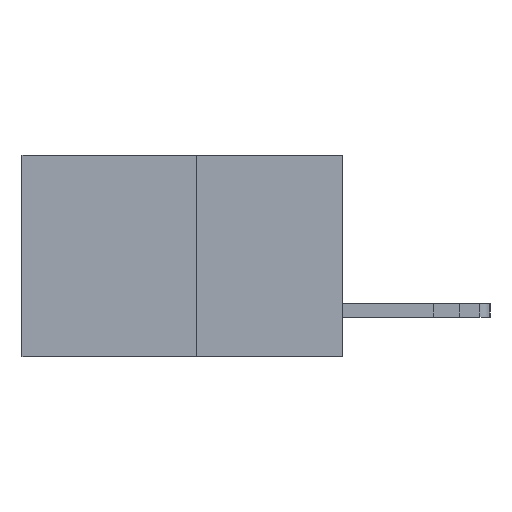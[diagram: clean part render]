
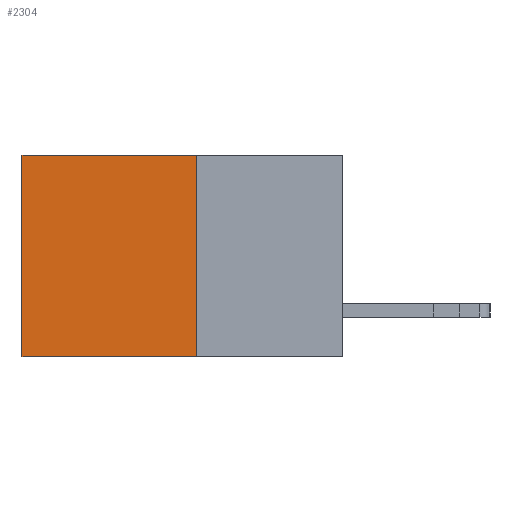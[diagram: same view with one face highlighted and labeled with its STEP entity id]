
A CAD part, left-side view. The second image highlights one B-rep face of the part: STEP entity #2304.
In plain terms, the highlighted planar face has unit normal (-1, 0, 0).
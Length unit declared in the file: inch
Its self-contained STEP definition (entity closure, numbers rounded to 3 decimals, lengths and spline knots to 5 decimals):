
#92 = EDGE_CURVE ( 'NONE', #1988, #14659, #19713, .T. ) ;
#217 = AXIS2_PLACEMENT_3D ( 'NONE', #9727, #699, #9771 ) ;
#699 = DIRECTION ( 'NONE',  ( 1., 0., 0. ) ) ;
#1071 = CARTESIAN_POINT ( 'NONE',  ( 0.277, 0.59, -0.37 ) ) ;
#1251 = EDGE_CURVE ( 'NONE', #15106, #1988, #3386, .T. ) ;
#1988 = VERTEX_POINT ( 'NONE', #11084 ) ;
#2304 = ADVANCED_FACE ( 'NONE', ( #20178 ), #7277, .F. ) ;
#2901 = VECTOR ( 'NONE', #3780, 39.37008 ) ;
#3386 = LINE ( 'NONE', #4396, #2901 ) ;
#3493 = DIRECTION ( 'NONE',  ( 0., 0., -1. ) ) ;
#3780 = DIRECTION ( 'NONE',  ( 0., 1., 0. ) ) ;
#4267 = CARTESIAN_POINT ( 'NONE',  ( 0.277, 0.27, -0.37 ) ) ;
#4396 = CARTESIAN_POINT ( 'NONE',  ( 0.277, 0.27, 0. ) ) ;
#4501 = LINE ( 'NONE', #12876, #5002 ) ;
#5002 = VECTOR ( 'NONE', #3493, 39.37008 ) ;
#6899 = ORIENTED_EDGE ( 'NONE', *, *, #92, .T. ) ;
#7020 = EDGE_CURVE ( 'NONE', #11213, #14659, #14625, .T. ) ;
#7277 = PLANE ( 'NONE',  #217 ) ;
#7416 = DIRECTION ( 'NONE',  ( 0., 0., -1. ) ) ;
#8427 = CARTESIAN_POINT ( 'NONE',  ( 0.277, 0.59, -0.37 ) ) ;
#9727 = CARTESIAN_POINT ( 'NONE',  ( 0.277, 0.27, -0.37 ) ) ;
#9771 = DIRECTION ( 'NONE',  ( 0., 0., -1. ) ) ;
#9920 = CARTESIAN_POINT ( 'NONE',  ( 0.277, 0.27, 0. ) ) ;
#11084 = CARTESIAN_POINT ( 'NONE',  ( 0.277, 0.59, 0. ) ) ;
#11213 = VERTEX_POINT ( 'NONE', #20085 ) ;
#11451 = ORIENTED_EDGE ( 'NONE', *, *, #13030, .F. ) ;
#11473 = VECTOR ( 'NONE', #7416, 39.37008 ) ;
#12876 = CARTESIAN_POINT ( 'NONE',  ( 0.277, 0.27, -0.37 ) ) ;
#13030 = EDGE_CURVE ( 'NONE', #15106, #11213, #4501, .T. ) ;
#13390 = ORIENTED_EDGE ( 'NONE', *, *, #7020, .F. ) ;
#13877 = ORIENTED_EDGE ( 'NONE', *, *, #1251, .T. ) ;
#14625 = LINE ( 'NONE', #4267, #17287 ) ;
#14659 = VERTEX_POINT ( 'NONE', #1071 ) ;
#15106 = VERTEX_POINT ( 'NONE', #9920 ) ;
#16537 = EDGE_LOOP ( 'NONE', ( #6899, #13390, #11451, #13877 ) ) ;
#17287 = VECTOR ( 'NONE', #18379, 39.37008 ) ;
#18379 = DIRECTION ( 'NONE',  ( 0., 1., 0. ) ) ;
#19713 = LINE ( 'NONE', #8427, #11473 ) ;
#20085 = CARTESIAN_POINT ( 'NONE',  ( 0.277, 0.27, -0.37 ) ) ;
#20178 = FACE_OUTER_BOUND ( 'NONE', #16537, .T. ) ;
